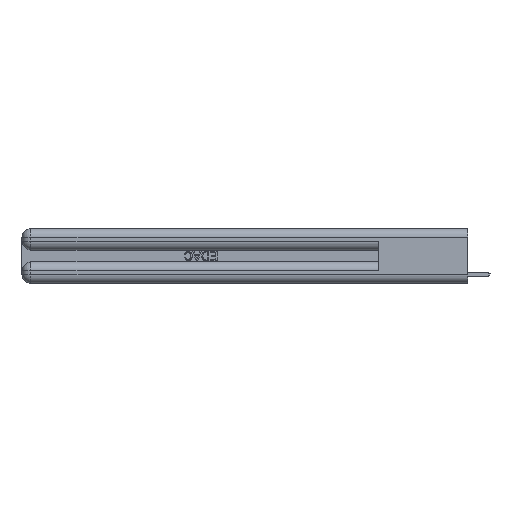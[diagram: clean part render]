
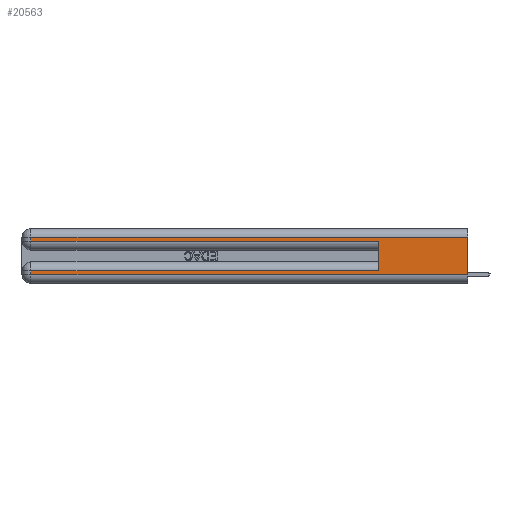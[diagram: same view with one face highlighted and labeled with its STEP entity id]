
A CAD part, left-side view. The second image highlights one B-rep face of the part: STEP entity #20563.
In plain terms, the highlighted planar face has unit normal (-1, 0, 0).
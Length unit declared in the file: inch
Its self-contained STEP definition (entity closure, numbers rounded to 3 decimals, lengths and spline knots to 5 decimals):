
#377 = VERTEX_POINT ( 'NONE', #13644 ) ;
#1397 = CARTESIAN_POINT ( 'NONE',  ( 0., 2.94, 0.285 ) ) ;
#1468 = VECTOR ( 'NONE', #14990, 39.37008 ) ;
#2210 = VECTOR ( 'NONE', #14569, 39.37008 ) ;
#2986 = LINE ( 'NONE', #29435, #34017 ) ;
#3208 = DIRECTION ( 'NONE',  ( 0., 0., 1. ) ) ;
#4054 = CARTESIAN_POINT ( 'NONE',  ( 0., 2.94, 0.37 ) ) ;
#4827 = LINE ( 'NONE', #18108, #12993 ) ;
#4870 = FACE_OUTER_BOUND ( 'NONE', #13176, .T. ) ;
#5345 = VERTEX_POINT ( 'NONE', #24939 ) ;
#5760 = VERTEX_POINT ( 'NONE', #1397 ) ;
#6060 = CARTESIAN_POINT ( 'NONE',  ( 0., 0.6, 0.085 ) ) ;
#6263 = CARTESIAN_POINT ( 'NONE',  ( 0., 2.94, 0.37 ) ) ;
#6399 = VECTOR ( 'NONE', #27320, 39.37008 ) ;
#8023 = VECTOR ( 'NONE', #21939, 39.37008 ) ;
#9685 = CARTESIAN_POINT ( 'NONE',  ( 0., 0., 0.37 ) ) ;
#10591 = EDGE_CURVE ( 'NONE', #22076, #25158, #19374, .T. ) ;
#10640 = EDGE_CURVE ( 'NONE', #25158, #377, #19891, .T. ) ;
#10904 = CARTESIAN_POINT ( 'NONE',  ( 0., 0., 0.31 ) ) ;
#11297 = EDGE_CURVE ( 'NONE', #377, #33298, #15656, .T. ) ;
#11383 = CARTESIAN_POINT ( 'NONE',  ( 0., 0., 0.31 ) ) ;
#12382 = ORIENTED_EDGE ( 'NONE', *, *, #32463, .F. ) ;
#12558 = DIRECTION ( 'NONE',  ( 0., -1., 0. ) ) ;
#12785 = DIRECTION ( 'NONE',  ( 0., 0., -1. ) ) ;
#12993 = VECTOR ( 'NONE', #3208, 39.37008 ) ;
#13176 = EDGE_LOOP ( 'NONE', ( #14759, #20282, #27980, #24932, #12382, #28781, #23374, #25264 ) ) ;
#13644 = CARTESIAN_POINT ( 'NONE',  ( 0., 2.94, 0.06 ) ) ;
#14569 = DIRECTION ( 'NONE',  ( 0., 0., -1. ) ) ;
#14759 = ORIENTED_EDGE ( 'NONE', *, *, #32845, .F. ) ;
#14990 = DIRECTION ( 'NONE',  ( 0., -1., 0. ) ) ;
#15656 = LINE ( 'NONE', #28831, #1468 ) ;
#16372 = EDGE_CURVE ( 'NONE', #5760, #21767, #28833, .T. ) ;
#17146 = EDGE_CURVE ( 'NONE', #5345, #5760, #19764, .T. ) ;
#17358 = VERTEX_POINT ( 'NONE', #10904 ) ;
#18108 = CARTESIAN_POINT ( 'NONE',  ( 0., 0.6, 0.145 ) ) ;
#18520 = DIRECTION ( 'NONE',  ( 0., 0., -1. ) ) ;
#19374 = LINE ( 'NONE', #32681, #30112 ) ;
#19764 = LINE ( 'NONE', #4054, #2210 ) ;
#19891 = LINE ( 'NONE', #6263, #6399 ) ;
#20282 = ORIENTED_EDGE ( 'NONE', *, *, #32287, .T. ) ;
#20287 = AXIS2_PLACEMENT_3D ( 'NONE', #9685, #23171, #12785 ) ;
#20563 = ADVANCED_FACE ( 'NONE', ( #4870 ), #20581, .F. ) ;
#20581 = PLANE ( 'NONE',  #20287 ) ;
#21767 = VERTEX_POINT ( 'NONE', #28034 ) ;
#21939 = DIRECTION ( 'NONE',  ( 0., 1., 0. ) ) ;
#22076 = VERTEX_POINT ( 'NONE', #6060 ) ;
#22125 = VECTOR ( 'NONE', #12558, 39.37008 ) ;
#23171 = DIRECTION ( 'NONE',  ( 1., 0., 0. ) ) ;
#23374 = ORIENTED_EDGE ( 'NONE', *, *, #10640, .T. ) ;
#24364 = CARTESIAN_POINT ( 'NONE',  ( 0., 0., 0.06 ) ) ;
#24528 = LINE ( 'NONE', #11383, #8023 ) ;
#24919 = CARTESIAN_POINT ( 'NONE',  ( 0., 2.94, 0.085 ) ) ;
#24932 = ORIENTED_EDGE ( 'NONE', *, *, #16372, .T. ) ;
#24939 = CARTESIAN_POINT ( 'NONE',  ( 0., 2.94, 0.31 ) ) ;
#25158 = VERTEX_POINT ( 'NONE', #24919 ) ;
#25264 = ORIENTED_EDGE ( 'NONE', *, *, #11297, .T. ) ;
#25698 = CARTESIAN_POINT ( 'NONE',  ( 0., 0., 0.285 ) ) ;
#27320 = DIRECTION ( 'NONE',  ( 0., 0., -1. ) ) ;
#27844 = DIRECTION ( 'NONE',  ( 0., 1., 0. ) ) ;
#27980 = ORIENTED_EDGE ( 'NONE', *, *, #17146, .T. ) ;
#28034 = CARTESIAN_POINT ( 'NONE',  ( 0., 0.6, 0.285 ) ) ;
#28781 = ORIENTED_EDGE ( 'NONE', *, *, #10591, .T. ) ;
#28831 = CARTESIAN_POINT ( 'NONE',  ( 0., 0., 0.06 ) ) ;
#28833 = LINE ( 'NONE', #25698, #22125 ) ;
#29435 = CARTESIAN_POINT ( 'NONE',  ( 0., 0., 0.37 ) ) ;
#30112 = VECTOR ( 'NONE', #27844, 39.37008 ) ;
#32287 = EDGE_CURVE ( 'NONE', #17358, #5345, #24528, .T. ) ;
#32463 = EDGE_CURVE ( 'NONE', #22076, #21767, #4827, .T. ) ;
#32681 = CARTESIAN_POINT ( 'NONE',  ( 0., 0., 0.085 ) ) ;
#32845 = EDGE_CURVE ( 'NONE', #17358, #33298, #2986, .T. ) ;
#33298 = VERTEX_POINT ( 'NONE', #24364 ) ;
#34017 = VECTOR ( 'NONE', #18520, 39.37008 ) ;
